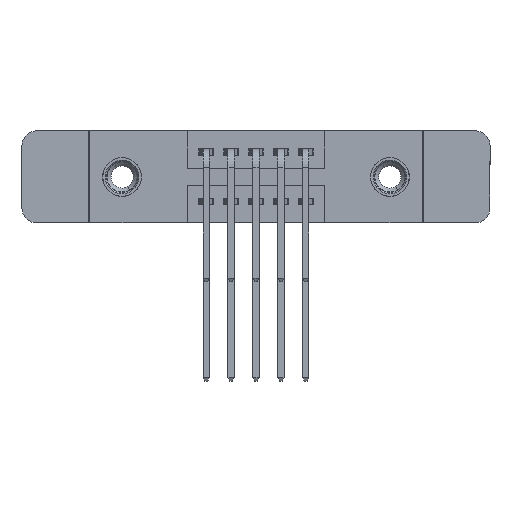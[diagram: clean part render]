
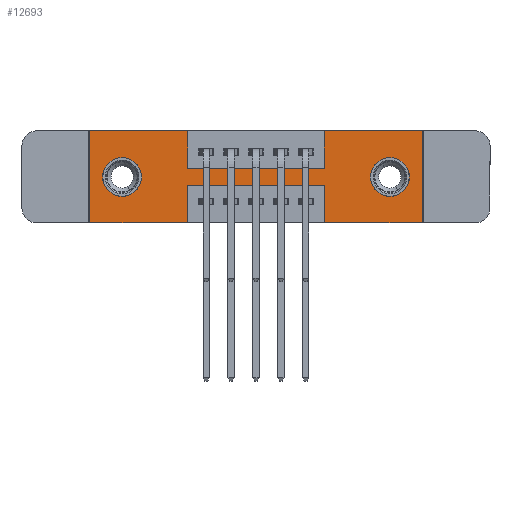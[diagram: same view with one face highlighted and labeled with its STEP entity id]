
A CAD part, front view. The second image highlights one B-rep face of the part: STEP entity #12693.
In plain terms, the highlighted planar face has unit normal (0, -1, 0).
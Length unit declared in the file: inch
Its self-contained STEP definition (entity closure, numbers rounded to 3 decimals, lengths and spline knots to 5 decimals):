
#48 = CARTESIAN_POINT ( 'NONE',  ( 0., 0., 0. ) ) ;
#71 = VERTEX_POINT ( 'NONE', #12917 ) ;
#96 = AXIS2_PLACEMENT_3D ( 'NONE', #6550, #7720, #11348 ) ;
#295 = EDGE_CURVE ( 'NONE', #7226, #12334, #5111, .T. ) ;
#356 = CARTESIAN_POINT ( 'NONE',  ( 1.205, 0., -0.185 ) ) ;
#405 = LINE ( 'NONE', #4340, #15607 ) ;
#548 = DIRECTION ( 'NONE',  ( 0., 0., 1. ) ) ;
#600 = DIRECTION ( 'NONE',  ( 0., 0., -1. ) ) ;
#745 = DIRECTION ( 'NONE',  ( 1., 0., 0. ) ) ;
#838 = VERTEX_POINT ( 'NONE', #10026 ) ;
#917 = CARTESIAN_POINT ( 'NONE',  ( 0.13, 0., -0.263 ) ) ;
#1005 = CARTESIAN_POINT ( 'NONE',  ( 1.335, 0., 0. ) ) ;
#1205 = EDGE_CURVE ( 'NONE', #71, #1998, #12701, .T. ) ;
#1261 = PLANE ( 'NONE',  #13544 ) ;
#1288 = CARTESIAN_POINT ( 'NONE',  ( 0., 0., -0.37 ) ) ;
#1347 = ORIENTED_EDGE ( 'NONE', *, *, #295, .F. ) ;
#1416 = LINE ( 'NONE', #8216, #3142 ) ;
#1473 = VERTEX_POINT ( 'NONE', #13427 ) ;
#1492 = EDGE_CURVE ( 'NONE', #1473, #838, #2792, .T. ) ;
#1854 = ORIENTED_EDGE ( 'NONE', *, *, #9576, .F. ) ;
#1892 = EDGE_CURVE ( 'NONE', #5076, #8180, #12690, .T. ) ;
#1937 = ORIENTED_EDGE ( 'NONE', *, *, #8184, .F. ) ;
#1957 = LINE ( 'NONE', #12909, #6005 ) ;
#1998 = VERTEX_POINT ( 'NONE', #4690 ) ;
#2053 = VERTEX_POINT ( 'NONE', #917 ) ;
#2073 = EDGE_CURVE ( 'NONE', #12334, #2360, #1416, .T. ) ;
#2129 = CARTESIAN_POINT ( 'NONE',  ( 0.3925, 0., 0. ) ) ;
#2257 = CARTESIAN_POINT ( 'NONE',  ( 0.3925, 0., -0.37 ) ) ;
#2278 = AXIS2_PLACEMENT_3D ( 'NONE', #9568, #5960, #4773 ) ;
#2306 = ORIENTED_EDGE ( 'NONE', *, *, #11569, .F. ) ;
#2360 = VERTEX_POINT ( 'NONE', #7902 ) ;
#2451 = CARTESIAN_POINT ( 'NONE',  ( 0.3925, 0., -0.22 ) ) ;
#2478 = AXIS2_PLACEMENT_3D ( 'NONE', #356, #13667, #11273 ) ;
#2486 = DIRECTION ( 'NONE',  ( 1., 0., 0. ) ) ;
#2541 = AXIS2_PLACEMENT_3D ( 'NONE', #10893, #8392, #4879 ) ;
#2686 = EDGE_LOOP ( 'NONE', ( #13316, #5320 ) ) ;
#2792 = LINE ( 'NONE', #14767, #13465 ) ;
#3049 = VERTEX_POINT ( 'NONE', #2451 ) ;
#3142 = VECTOR ( 'NONE', #10666, 39.37008 ) ;
#3150 = ORIENTED_EDGE ( 'NONE', *, *, #1492, .F. ) ;
#3192 = CARTESIAN_POINT ( 'NONE',  ( 1.335, 0., -0.37 ) ) ;
#3229 = VECTOR ( 'NONE', #745, 39.37008 ) ;
#3231 = EDGE_CURVE ( 'NONE', #12761, #2053, #8755, .T. ) ;
#3318 = ORIENTED_EDGE ( 'NONE', *, *, #13184, .F. ) ;
#3399 = DIRECTION ( 'NONE',  ( -1., 0., 0. ) ) ;
#3519 = ORIENTED_EDGE ( 'NONE', *, *, #5215, .F. ) ;
#3762 = CARTESIAN_POINT ( 'NONE',  ( 0., 0., 0. ) ) ;
#3825 = CIRCLE ( 'NONE', #2478, 0.078 ) ;
#3862 = CARTESIAN_POINT ( 'NONE',  ( 0.9425, 0., 0. ) ) ;
#4335 = LINE ( 'NONE', #13137, #8902 ) ;
#4340 = CARTESIAN_POINT ( 'NONE',  ( 0.9425, 0., 0. ) ) ;
#4485 = ORIENTED_EDGE ( 'NONE', *, *, #4767, .F. ) ;
#4690 = CARTESIAN_POINT ( 'NONE',  ( 1.205, 0., -0.107 ) ) ;
#4754 = VERTEX_POINT ( 'NONE', #3862 ) ;
#4767 = EDGE_CURVE ( 'NONE', #6494, #5076, #12126, .T. ) ;
#4773 = DIRECTION ( 'NONE',  ( 0., 0., 1. ) ) ;
#4840 = ORIENTED_EDGE ( 'NONE', *, *, #13067, .F. ) ;
#4877 = VECTOR ( 'NONE', #8103, 39.37008 ) ;
#4879 = DIRECTION ( 'NONE',  ( 0., 0., 1. ) ) ;
#4888 = DIRECTION ( 'NONE',  ( -1., 0., 0. ) ) ;
#4896 = CARTESIAN_POINT ( 'NONE',  ( 0.9425, 0., -0.22 ) ) ;
#5076 = VERTEX_POINT ( 'NONE', #48 ) ;
#5080 = CARTESIAN_POINT ( 'NONE',  ( 0.3925, 0., -0.37 ) ) ;
#5111 = LINE ( 'NONE', #5458, #11190 ) ;
#5215 = EDGE_CURVE ( 'NONE', #8180, #1473, #8102, .T. ) ;
#5226 = CARTESIAN_POINT ( 'NONE',  ( 0.13, 0., -0.107 ) ) ;
#5320 = ORIENTED_EDGE ( 'NONE', *, *, #1205, .T. ) ;
#5336 = ORIENTED_EDGE ( 'NONE', *, *, #1892, .F. ) ;
#5458 = CARTESIAN_POINT ( 'NONE',  ( 1.335, 0., 0. ) ) ;
#5497 = FACE_OUTER_BOUND ( 'NONE', #11989, .T. ) ;
#5659 = CARTESIAN_POINT ( 'NONE',  ( 0., 0., 0. ) ) ;
#5744 = CARTESIAN_POINT ( 'NONE',  ( 0.3925, 0., 0. ) ) ;
#5960 = DIRECTION ( 'NONE',  ( 0., 1., 0. ) ) ;
#5992 = EDGE_CURVE ( 'NONE', #2360, #7846, #1957, .T. ) ;
#6005 = VECTOR ( 'NONE', #548, 39.37008 ) ;
#6202 = CARTESIAN_POINT ( 'NONE',  ( 0., 0., -0.37 ) ) ;
#6253 = VERTEX_POINT ( 'NONE', #2257 ) ;
#6484 = LINE ( 'NONE', #5659, #3229 ) ;
#6494 = VERTEX_POINT ( 'NONE', #1288 ) ;
#6550 = CARTESIAN_POINT ( 'NONE',  ( 1.205, 0., -0.185 ) ) ;
#6631 = FACE_BOUND ( 'NONE', #14676, .T. ) ;
#6795 = VECTOR ( 'NONE', #2486, 39.37008 ) ;
#6926 = CIRCLE ( 'NONE', #2541, 0.078 ) ;
#7226 = VERTEX_POINT ( 'NONE', #1005 ) ;
#7292 = DIRECTION ( 'NONE',  ( 0., 0., 1. ) ) ;
#7409 = DIRECTION ( 'NONE',  ( 0., 0., -1. ) ) ;
#7427 = LINE ( 'NONE', #5080, #14073 ) ;
#7720 = DIRECTION ( 'NONE',  ( 0., 1., 0. ) ) ;
#7846 = VERTEX_POINT ( 'NONE', #4896 ) ;
#7902 = CARTESIAN_POINT ( 'NONE',  ( 0.9425, 0., -0.37 ) ) ;
#7931 = EDGE_CURVE ( 'NONE', #1998, #71, #3825, .T. ) ;
#8102 = LINE ( 'NONE', #2129, #4877 ) ;
#8103 = DIRECTION ( 'NONE',  ( 0., 0., -1. ) ) ;
#8180 = VERTEX_POINT ( 'NONE', #5744 ) ;
#8184 = EDGE_CURVE ( 'NONE', #838, #4754, #405, .T. ) ;
#8216 = CARTESIAN_POINT ( 'NONE',  ( 0., 0., -0.37 ) ) ;
#8392 = DIRECTION ( 'NONE',  ( 0., 1., 0. ) ) ;
#8616 = ORIENTED_EDGE ( 'NONE', *, *, #15611, .T. ) ;
#8719 = LINE ( 'NONE', #10954, #14038 ) ;
#8755 = CIRCLE ( 'NONE', #2278, 0.078 ) ;
#8902 = VECTOR ( 'NONE', #3399, 39.37008 ) ;
#9568 = CARTESIAN_POINT ( 'NONE',  ( 0.13, 0., -0.185 ) ) ;
#9576 = EDGE_CURVE ( 'NONE', #3049, #6253, #7427, .T. ) ;
#10026 = CARTESIAN_POINT ( 'NONE',  ( 0.9425, 0., -0.15 ) ) ;
#10344 = ORIENTED_EDGE ( 'NONE', *, *, #3231, .T. ) ;
#10666 = DIRECTION ( 'NONE',  ( -1., 0., 0. ) ) ;
#10893 = CARTESIAN_POINT ( 'NONE',  ( 0.13, 0., -0.185 ) ) ;
#10954 = CARTESIAN_POINT ( 'NONE',  ( 0.3925, 0., -0.22 ) ) ;
#11164 = CARTESIAN_POINT ( 'NONE',  ( 0., 0., 0. ) ) ;
#11190 = VECTOR ( 'NONE', #600, 39.37008 ) ;
#11273 = DIRECTION ( 'NONE',  ( 0., 0., -1. ) ) ;
#11348 = DIRECTION ( 'NONE',  ( 0., 0., -1. ) ) ;
#11569 = EDGE_CURVE ( 'NONE', #4754, #7226, #6484, .T. ) ;
#11989 = EDGE_LOOP ( 'NONE', ( #1854, #3318, #13446, #13420, #1347, #2306, #1937, #3150, #3519, #5336, #4485, #4840 ) ) ;
#12126 = LINE ( 'NONE', #11164, #12702 ) ;
#12308 = DIRECTION ( 'NONE',  ( 0., 0., -1. ) ) ;
#12334 = VERTEX_POINT ( 'NONE', #3192 ) ;
#12690 = LINE ( 'NONE', #3762, #6795 ) ;
#12693 = ADVANCED_FACE ( 'NONE', ( #15168, #6631, #5497 ), #1261, .T. ) ;
#12701 = CIRCLE ( 'NONE', #96, 0.078 ) ;
#12702 = VECTOR ( 'NONE', #7292, 39.37008 ) ;
#12761 = VERTEX_POINT ( 'NONE', #5226 ) ;
#12909 = CARTESIAN_POINT ( 'NONE',  ( 0.9425, 0., -0.37 ) ) ;
#12917 = CARTESIAN_POINT ( 'NONE',  ( 1.205, 0., -0.263 ) ) ;
#13067 = EDGE_CURVE ( 'NONE', #6253, #6494, #4335, .T. ) ;
#13137 = CARTESIAN_POINT ( 'NONE',  ( 0., 0., -0.37 ) ) ;
#13184 = EDGE_CURVE ( 'NONE', #7846, #3049, #8719, .T. ) ;
#13316 = ORIENTED_EDGE ( 'NONE', *, *, #7931, .T. ) ;
#13420 = ORIENTED_EDGE ( 'NONE', *, *, #2073, .F. ) ;
#13427 = CARTESIAN_POINT ( 'NONE',  ( 0.3925, 0., -0.15 ) ) ;
#13446 = ORIENTED_EDGE ( 'NONE', *, *, #5992, .F. ) ;
#13465 = VECTOR ( 'NONE', #14219, 39.37008 ) ;
#13544 = AXIS2_PLACEMENT_3D ( 'NONE', #6202, #14680, #7409 ) ;
#13667 = DIRECTION ( 'NONE',  ( 0., 1., 0. ) ) ;
#14038 = VECTOR ( 'NONE', #4888, 39.37008 ) ;
#14073 = VECTOR ( 'NONE', #12308, 39.37008 ) ;
#14219 = DIRECTION ( 'NONE',  ( 1., 0., 0. ) ) ;
#14676 = EDGE_LOOP ( 'NONE', ( #10344, #8616 ) ) ;
#14680 = DIRECTION ( 'NONE',  ( 0., -1., 0. ) ) ;
#14767 = CARTESIAN_POINT ( 'NONE',  ( 0.3925, 0., -0.15 ) ) ;
#15168 = FACE_BOUND ( 'NONE', #2686, .T. ) ;
#15224 = DIRECTION ( 'NONE',  ( 0., 0., 1. ) ) ;
#15607 = VECTOR ( 'NONE', #15224, 39.37008 ) ;
#15611 = EDGE_CURVE ( 'NONE', #2053, #12761, #6926, .T. ) ;
